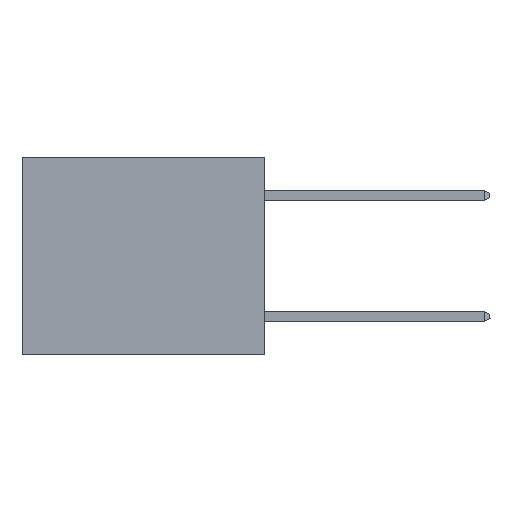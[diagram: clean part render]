
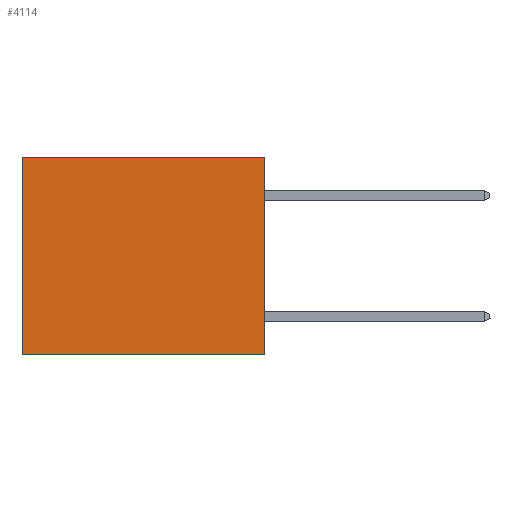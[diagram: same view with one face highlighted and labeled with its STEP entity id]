
A CAD part, left-side view. The second image highlights one B-rep face of the part: STEP entity #4114.
In plain terms, the highlighted planar face has unit normal (-1, 0, 0).
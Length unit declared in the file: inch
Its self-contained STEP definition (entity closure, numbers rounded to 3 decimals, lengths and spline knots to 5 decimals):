
#775 = LINE ( 'NONE', #13283, #12486 ) ;
#1024 = EDGE_CURVE ( 'NONE', #11416, #2476, #775, .T. ) ;
#1376 = EDGE_CURVE ( 'NONE', #17038, #11416, #7738, .T. ) ;
#2476 = VERTEX_POINT ( 'NONE', #13622 ) ;
#3362 = CARTESIAN_POINT ( 'NONE',  ( 0.3165, 0., -0.49 ) ) ;
#4114 = ADVANCED_FACE ( 'NONE', ( #6103 ), #13269, .F. ) ;
#4997 = DIRECTION ( 'NONE',  ( 0., 0., -1. ) ) ;
#5305 = EDGE_CURVE ( 'NONE', #17038, #8732, #17992, .T. ) ;
#5372 = CARTESIAN_POINT ( 'NONE',  ( 0.3165, 0., -0.49 ) ) ;
#6008 = EDGE_LOOP ( 'NONE', ( #11167, #19810, #19363, #18097 ) ) ;
#6103 = FACE_OUTER_BOUND ( 'NONE', #6008, .T. ) ;
#6308 = VECTOR ( 'NONE', #6401, 39.37008 ) ;
#6401 = DIRECTION ( 'NONE',  ( 0., 1., 0. ) ) ;
#6441 = EDGE_CURVE ( 'NONE', #8732, #2476, #10712, .T. ) ;
#6500 = VECTOR ( 'NONE', #19708, 39.37008 ) ;
#7738 = LINE ( 'NONE', #5372, #6500 ) ;
#8557 = DIRECTION ( 'NONE',  ( 1., 0., 0. ) ) ;
#8732 = VERTEX_POINT ( 'NONE', #13748 ) ;
#9483 = VECTOR ( 'NONE', #4997, 39.37008 ) ;
#10712 = LINE ( 'NONE', #13155, #9483 ) ;
#11167 = ORIENTED_EDGE ( 'NONE', *, *, #6441, .T. ) ;
#11416 = VERTEX_POINT ( 'NONE', #3362 ) ;
#12486 = VECTOR ( 'NONE', #19555, 39.37008 ) ;
#12640 = CARTESIAN_POINT ( 'NONE',  ( 0.3165, 0., 0. ) ) ;
#13155 = CARTESIAN_POINT ( 'NONE',  ( 0.3165, 0.6, -0.49 ) ) ;
#13269 = PLANE ( 'NONE',  #19353 ) ;
#13283 = CARTESIAN_POINT ( 'NONE',  ( 0.3165, 0., -0.49 ) ) ;
#13335 = CARTESIAN_POINT ( 'NONE',  ( 0.3165, 0., -0.49 ) ) ;
#13622 = CARTESIAN_POINT ( 'NONE',  ( 0.3165, 0.6, -0.49 ) ) ;
#13748 = CARTESIAN_POINT ( 'NONE',  ( 0.3165, 0.6, 0. ) ) ;
#14778 = DIRECTION ( 'NONE',  ( 0., 0., -1. ) ) ;
#17038 = VERTEX_POINT ( 'NONE', #19993 ) ;
#17992 = LINE ( 'NONE', #12640, #6308 ) ;
#18097 = ORIENTED_EDGE ( 'NONE', *, *, #5305, .T. ) ;
#19353 = AXIS2_PLACEMENT_3D ( 'NONE', #13335, #8557, #14778 ) ;
#19363 = ORIENTED_EDGE ( 'NONE', *, *, #1376, .F. ) ;
#19555 = DIRECTION ( 'NONE',  ( 0., 1., 0. ) ) ;
#19708 = DIRECTION ( 'NONE',  ( 0., 0., -1. ) ) ;
#19810 = ORIENTED_EDGE ( 'NONE', *, *, #1024, .F. ) ;
#19993 = CARTESIAN_POINT ( 'NONE',  ( 0.3165, 0., 0. ) ) ;
